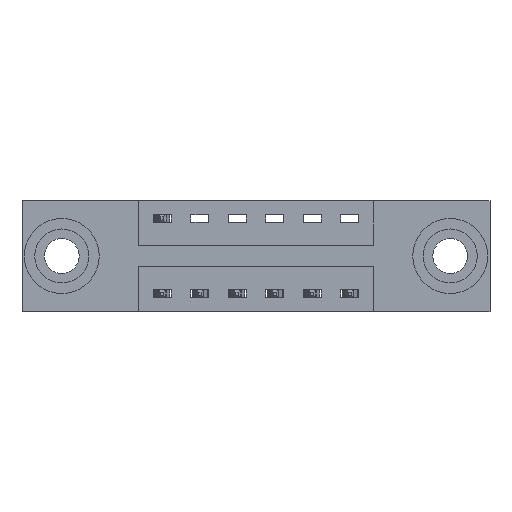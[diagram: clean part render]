
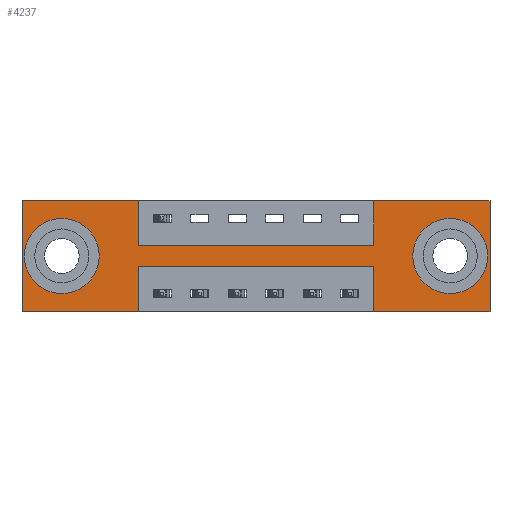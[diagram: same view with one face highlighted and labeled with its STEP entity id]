
A CAD part, front view. The second image highlights one B-rep face of the part: STEP entity #4237.
In plain terms, the highlighted planar face has unit normal (0, -1, 0).
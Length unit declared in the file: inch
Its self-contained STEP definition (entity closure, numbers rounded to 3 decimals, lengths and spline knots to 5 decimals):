
#85 = CARTESIAN_POINT ( 'NONE',  ( 0., 0., -0.37 ) ) ;
#86 = CARTESIAN_POINT ( 'NONE',  ( 1.56, 0., -0.37 ) ) ;
#90 = ORIENTED_EDGE ( 'NONE', *, *, #2126, .F. ) ;
#186 = ORIENTED_EDGE ( 'NONE', *, *, #5030, .F. ) ;
#219 = EDGE_CURVE ( 'NONE', #7737, #376, #1409, .T. ) ;
#364 = ORIENTED_EDGE ( 'NONE', *, *, #1254, .F. ) ;
#376 = VERTEX_POINT ( 'NONE', #9186 ) ;
#428 = LINE ( 'NONE', #6002, #5897 ) ;
#479 = CARTESIAN_POINT ( 'NONE',  ( 1.1725, 0., -0.37 ) ) ;
#1154 = ORIENTED_EDGE ( 'NONE', *, *, #219, .F. ) ;
#1221 = DIRECTION ( 'NONE',  ( 1., 0., 0. ) ) ;
#1254 = EDGE_CURVE ( 'NONE', #7412, #1300, #8044, .T. ) ;
#1263 = DIRECTION ( 'NONE',  ( 1., 0., 0. ) ) ;
#1286 = ORIENTED_EDGE ( 'NONE', *, *, #9105, .F. ) ;
#1300 = VERTEX_POINT ( 'NONE', #7047 ) ;
#1370 = DIRECTION ( 'NONE',  ( 0., 0., 1. ) ) ;
#1394 = DIRECTION ( 'NONE',  ( 0., 1., 0. ) ) ;
#1396 = VERTEX_POINT ( 'NONE', #8186 ) ;
#1407 = CARTESIAN_POINT ( 'NONE',  ( 0.1325, 0., -0.185 ) ) ;
#1409 = LINE ( 'NONE', #4302, #8527 ) ;
#1482 = AXIS2_PLACEMENT_3D ( 'NONE', #7816, #7805, #7803 ) ;
#1762 = AXIS2_PLACEMENT_3D ( 'NONE', #2386, #7226, #7212 ) ;
#1801 = VERTEX_POINT ( 'NONE', #4685 ) ;
#1881 = ORIENTED_EDGE ( 'NONE', *, *, #8564, .F. ) ;
#2058 = LINE ( 'NONE', #7769, #5595 ) ;
#2126 = EDGE_CURVE ( 'NONE', #5001, #7412, #4582, .T. ) ;
#2186 = FACE_BOUND ( 'NONE', #7526, .T. ) ;
#2191 = CARTESIAN_POINT ( 'NONE',  ( 0.1325, 0., -0.263 ) ) ;
#2210 = ORIENTED_EDGE ( 'NONE', *, *, #2843, .F. ) ;
#2349 = VECTOR ( 'NONE', #6336, 39.37008 ) ;
#2386 = CARTESIAN_POINT ( 'NONE',  ( 1.4275, 0., -0.185 ) ) ;
#2551 = DIRECTION ( 'NONE',  ( 0., 0., -1. ) ) ;
#2571 = CARTESIAN_POINT ( 'NONE',  ( 1.56, 0., 0. ) ) ;
#2624 = CARTESIAN_POINT ( 'NONE',  ( 1.1725, 0., 0. ) ) ;
#2662 = CARTESIAN_POINT ( 'NONE',  ( 0., 0., 0. ) ) ;
#2680 = CARTESIAN_POINT ( 'NONE',  ( 0.1325, 0., -0.107 ) ) ;
#2754 = ORIENTED_EDGE ( 'NONE', *, *, #5681, .F. ) ;
#2775 = LINE ( 'NONE', #5637, #2349 ) ;
#2780 = VERTEX_POINT ( 'NONE', #8359 ) ;
#2795 = CIRCLE ( 'NONE', #1762, 0.078 ) ;
#2813 = CARTESIAN_POINT ( 'NONE',  ( 0., 0., 0. ) ) ;
#2843 = EDGE_CURVE ( 'NONE', #1396, #7737, #428, .T. ) ;
#2845 = AXIS2_PLACEMENT_3D ( 'NONE', #8075, #3825, #3874 ) ;
#3039 = LINE ( 'NONE', #8365, #6782 ) ;
#3052 = VECTOR ( 'NONE', #3224, 39.37008 ) ;
#3067 = DIRECTION ( 'NONE',  ( 0., 1., 0. ) ) ;
#3220 = ORIENTED_EDGE ( 'NONE', *, *, #3656, .T. ) ;
#3224 = DIRECTION ( 'NONE',  ( 0., 0., -1. ) ) ;
#3279 = CARTESIAN_POINT ( 'NONE',  ( 0.3875, 0., 0. ) ) ;
#3323 = VECTOR ( 'NONE', #1263, 39.37008 ) ;
#3462 = EDGE_CURVE ( 'NONE', #7783, #7983, #4554, .T. ) ;
#3543 = LINE ( 'NONE', #2662, #3323 ) ;
#3559 = LINE ( 'NONE', #2571, #9034 ) ;
#3656 = EDGE_CURVE ( 'NONE', #9294, #4756, #2795, .T. ) ;
#3789 = EDGE_CURVE ( 'NONE', #376, #8706, #3559, .T. ) ;
#3803 = VERTEX_POINT ( 'NONE', #479 ) ;
#3825 = DIRECTION ( 'NONE',  ( 0., -1., 0. ) ) ;
#3868 = ORIENTED_EDGE ( 'NONE', *, *, #3462, .T. ) ;
#3874 = DIRECTION ( 'NONE',  ( 0., 0., -1. ) ) ;
#3946 = CARTESIAN_POINT ( 'NONE',  ( 0., 0., -0.37 ) ) ;
#3977 = DIRECTION ( 'NONE',  ( -1., 0., 0. ) ) ;
#4019 = VECTOR ( 'NONE', #4614, 39.37008 ) ;
#4033 = FACE_OUTER_BOUND ( 'NONE', #5203, .T. ) ;
#4061 = CARTESIAN_POINT ( 'NONE',  ( 0.3875, 0., -0.37 ) ) ;
#4080 = ORIENTED_EDGE ( 'NONE', *, *, #8763, .T. ) ;
#4237 = ADVANCED_FACE ( 'NONE', ( #4263, #2186, #4033 ), #8108, .T. ) ;
#4263 = FACE_BOUND ( 'NONE', #7376, .T. ) ;
#4276 = CARTESIAN_POINT ( 'NONE',  ( 1.4275, 0., -0.263 ) ) ;
#4302 = CARTESIAN_POINT ( 'NONE',  ( 0., 0., 0. ) ) ;
#4391 = VERTEX_POINT ( 'NONE', #7862 ) ;
#4554 = CIRCLE ( 'NONE', #4784, 0.078 ) ;
#4582 = LINE ( 'NONE', #9066, #8150 ) ;
#4614 = DIRECTION ( 'NONE',  ( 0., 0., 1. ) ) ;
#4685 = CARTESIAN_POINT ( 'NONE',  ( 0.3875, 0., -0.15 ) ) ;
#4756 = VERTEX_POINT ( 'NONE', #6497 ) ;
#4784 = AXIS2_PLACEMENT_3D ( 'NONE', #1407, #1394, #1370 ) ;
#4873 = ORIENTED_EDGE ( 'NONE', *, *, #5660, .T. ) ;
#5001 = VERTEX_POINT ( 'NONE', #4061 ) ;
#5030 = EDGE_CURVE ( 'NONE', #8706, #3803, #7239, .T. ) ;
#5078 = EDGE_CURVE ( 'NONE', #7446, #1801, #5369, .T. ) ;
#5203 = EDGE_LOOP ( 'NONE', ( #5614, #1881, #7868, #186, #6425, #1154, #2210, #2754, #5576, #1286, #364, #90 ) ) ;
#5369 = LINE ( 'NONE', #3279, #3052 ) ;
#5533 = EDGE_CURVE ( 'NONE', #3803, #4391, #3039, .T. ) ;
#5576 = ORIENTED_EDGE ( 'NONE', *, *, #5078, .F. ) ;
#5595 = VECTOR ( 'NONE', #7735, 39.37008 ) ;
#5614 = ORIENTED_EDGE ( 'NONE', *, *, #7736, .F. ) ;
#5637 = CARTESIAN_POINT ( 'NONE',  ( 0.3875, 0., -0.22 ) ) ;
#5660 = EDGE_CURVE ( 'NONE', #4756, #9294, #7799, .T. ) ;
#5681 = EDGE_CURVE ( 'NONE', #1801, #1396, #2058, .T. ) ;
#5844 = DIRECTION ( 'NONE',  ( 0., 0., 1. ) ) ;
#5861 = CARTESIAN_POINT ( 'NONE',  ( 0.3875, 0., 0. ) ) ;
#5897 = VECTOR ( 'NONE', #5844, 39.37008 ) ;
#6002 = CARTESIAN_POINT ( 'NONE',  ( 1.1725, 0., 0. ) ) ;
#6336 = DIRECTION ( 'NONE',  ( -1., 0., 0. ) ) ;
#6409 = CIRCLE ( 'NONE', #6818, 0.078 ) ;
#6425 = ORIENTED_EDGE ( 'NONE', *, *, #3789, .F. ) ;
#6497 = CARTESIAN_POINT ( 'NONE',  ( 1.4275, 0., -0.107 ) ) ;
#6782 = VECTOR ( 'NONE', #8352, 39.37008 ) ;
#6818 = AXIS2_PLACEMENT_3D ( 'NONE', #7288, #3067, #8031 ) ;
#6839 = CARTESIAN_POINT ( 'NONE',  ( 0.3875, 0., -0.37 ) ) ;
#6867 = VECTOR ( 'NONE', #7567, 39.37008 ) ;
#7047 = CARTESIAN_POINT ( 'NONE',  ( 0., 0., 0. ) ) ;
#7092 = LINE ( 'NONE', #6839, #6867 ) ;
#7212 = DIRECTION ( 'NONE',  ( 0., 0., -1. ) ) ;
#7226 = DIRECTION ( 'NONE',  ( 0., 1., 0. ) ) ;
#7239 = LINE ( 'NONE', #3946, #9180 ) ;
#7288 = CARTESIAN_POINT ( 'NONE',  ( 0.1325, 0., -0.185 ) ) ;
#7376 = EDGE_LOOP ( 'NONE', ( #4873, #3220 ) ) ;
#7412 = VERTEX_POINT ( 'NONE', #85 ) ;
#7446 = VERTEX_POINT ( 'NONE', #5861 ) ;
#7526 = EDGE_LOOP ( 'NONE', ( #3868, #4080 ) ) ;
#7567 = DIRECTION ( 'NONE',  ( 0., 0., -1. ) ) ;
#7735 = DIRECTION ( 'NONE',  ( 1., 0., 0. ) ) ;
#7736 = EDGE_CURVE ( 'NONE', #2780, #5001, #7092, .T. ) ;
#7737 = VERTEX_POINT ( 'NONE', #2624 ) ;
#7769 = CARTESIAN_POINT ( 'NONE',  ( 0.3875, 0., -0.15 ) ) ;
#7783 = VERTEX_POINT ( 'NONE', #2680 ) ;
#7799 = CIRCLE ( 'NONE', #1482, 0.078 ) ;
#7803 = DIRECTION ( 'NONE',  ( 0., 0., -1. ) ) ;
#7805 = DIRECTION ( 'NONE',  ( 0., 1., 0. ) ) ;
#7816 = CARTESIAN_POINT ( 'NONE',  ( 1.4275, 0., -0.185 ) ) ;
#7862 = CARTESIAN_POINT ( 'NONE',  ( 1.1725, 0., -0.22 ) ) ;
#7868 = ORIENTED_EDGE ( 'NONE', *, *, #5533, .F. ) ;
#7983 = VERTEX_POINT ( 'NONE', #2191 ) ;
#8031 = DIRECTION ( 'NONE',  ( 0., 0., 1. ) ) ;
#8044 = LINE ( 'NONE', #2813, #4019 ) ;
#8075 = CARTESIAN_POINT ( 'NONE',  ( 0., 0., -0.37 ) ) ;
#8108 = PLANE ( 'NONE',  #2845 ) ;
#8150 = VECTOR ( 'NONE', #9099, 39.37008 ) ;
#8186 = CARTESIAN_POINT ( 'NONE',  ( 1.1725, 0., -0.15 ) ) ;
#8352 = DIRECTION ( 'NONE',  ( 0., 0., 1. ) ) ;
#8359 = CARTESIAN_POINT ( 'NONE',  ( 0.3875, 0., -0.22 ) ) ;
#8365 = CARTESIAN_POINT ( 'NONE',  ( 1.1725, 0., -0.37 ) ) ;
#8527 = VECTOR ( 'NONE', #1221, 39.37008 ) ;
#8564 = EDGE_CURVE ( 'NONE', #4391, #2780, #2775, .T. ) ;
#8706 = VERTEX_POINT ( 'NONE', #86 ) ;
#8763 = EDGE_CURVE ( 'NONE', #7983, #7783, #6409, .T. ) ;
#9034 = VECTOR ( 'NONE', #2551, 39.37008 ) ;
#9066 = CARTESIAN_POINT ( 'NONE',  ( 0., 0., -0.37 ) ) ;
#9099 = DIRECTION ( 'NONE',  ( -1., 0., 0. ) ) ;
#9105 = EDGE_CURVE ( 'NONE', #1300, #7446, #3543, .T. ) ;
#9180 = VECTOR ( 'NONE', #3977, 39.37008 ) ;
#9186 = CARTESIAN_POINT ( 'NONE',  ( 1.56, 0., 0. ) ) ;
#9294 = VERTEX_POINT ( 'NONE', #4276 ) ;
